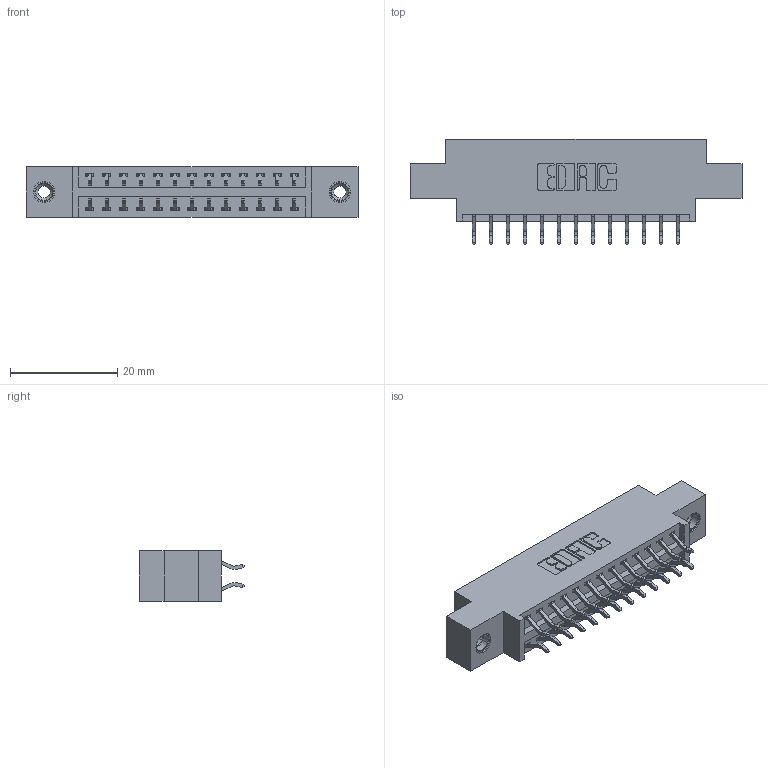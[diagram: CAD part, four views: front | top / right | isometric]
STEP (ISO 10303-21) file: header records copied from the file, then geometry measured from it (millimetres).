
FILE_DESCRIPTION (( 'STEP AP203' ), '1' );
FILE_NAME ('346-026-556-808.STEP', '2022-05-19T02:36:33', ( '' ), ( '' ), 'SwSTEP 2.0', 'SolidWorks 2020', '' );
FILE_SCHEMA (( 'CONFIG_CONTROL_DESIGN' ));
Length unit declared in the file: inch
Products named in the file (4): 346 Part_0.170 Offset - 0.156 Dia-TI; 346-026-556-808; 345-292-001_556 Tail; 345-250-001_345-250-003-102
Assembly tree (29 placements, depth 2):
  346-026-556-808
    346 Part_0.170 Offset - 0.156 Dia-TI
    345-292-001_556 Tail  x26
    345-250-001_345-250-003-102  x2
Bounding box: 61.85 x 19.57 x 9.4 mm (x, y, z)
Volume: 5643.7 mm3; surface area: 7477.3 mm2
Topology: 29 solids, 29 shells, 1694 faces, 4975 edges, 3274 vertices
Faces by surface type: plane 1126, cylinder 552, cone 12, torus 4
Entity records: 13926 total; most frequent: CARTESIAN_POINT 2335, ORIENTED_EDGE 2250, DIRECTION 2123, EDGE_CURVE 1125, VECTOR 913, LINE 913, VERTEX_POINT 744, AXIS2_PLACEMENT_3D 605
